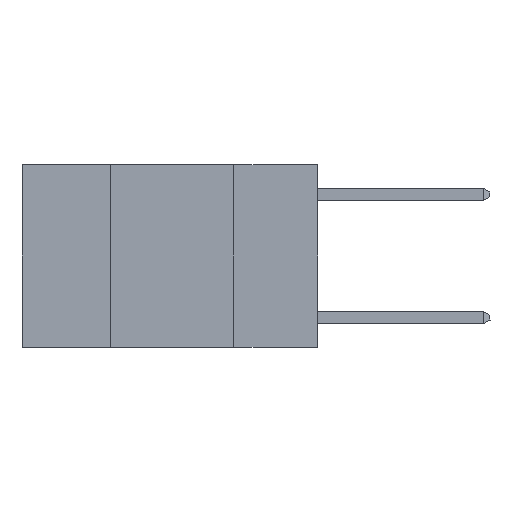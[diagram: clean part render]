
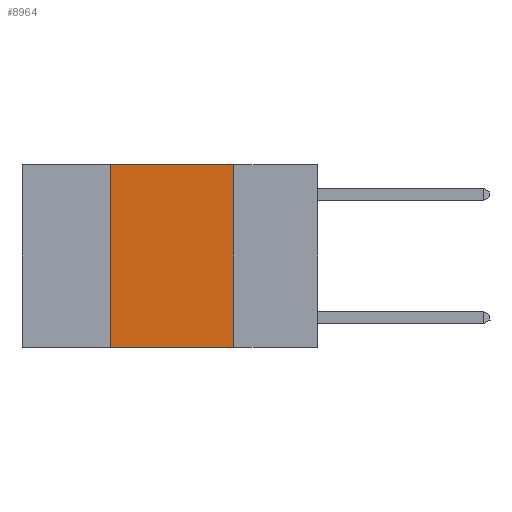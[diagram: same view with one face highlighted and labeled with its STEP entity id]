
A CAD part, left-side view. The second image highlights one B-rep face of the part: STEP entity #8964.
In plain terms, the highlighted planar face has unit normal (-1, 0, 0).
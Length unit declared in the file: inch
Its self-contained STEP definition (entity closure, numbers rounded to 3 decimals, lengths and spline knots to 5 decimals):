
#410 = VECTOR ( 'NONE', #20611, 39.37008 ) ;
#886 = CARTESIAN_POINT ( 'NONE',  ( 0., 0.42, 0. ) ) ;
#2584 = PLANE ( 'NONE',  #5424 ) ;
#3542 = VERTEX_POINT ( 'NONE', #16980 ) ;
#3792 = ORIENTED_EDGE ( 'NONE', *, *, #15846, .F. ) ;
#4309 = ORIENTED_EDGE ( 'NONE', *, *, #14849, .F. ) ;
#4364 = ORIENTED_EDGE ( 'NONE', *, *, #19608, .F. ) ;
#4509 = EDGE_LOOP ( 'NONE', ( #3792, #4309, #4364, #4764 ) ) ;
#4635 = CARTESIAN_POINT ( 'NONE',  ( 0., 0.6, 0. ) ) ;
#4764 = ORIENTED_EDGE ( 'NONE', *, *, #20805, .T. ) ;
#5039 = LINE ( 'NONE', #11954, #9811 ) ;
#5085 = VERTEX_POINT ( 'NONE', #16640 ) ;
#5424 = AXIS2_PLACEMENT_3D ( 'NONE', #4635, #18350, #6670 ) ;
#5779 = LINE ( 'NONE', #15813, #15697 ) ;
#6670 = DIRECTION ( 'NONE',  ( 0., 0., -1. ) ) ;
#6829 = VERTEX_POINT ( 'NONE', #14245 ) ;
#7136 = CARTESIAN_POINT ( 'NONE',  ( 0., 0.6, 0. ) ) ;
#8964 = ADVANCED_FACE ( 'NONE', ( #15971 ), #2584, .F. ) ;
#9811 = VECTOR ( 'NONE', #17681, 39.37008 ) ;
#10138 = DIRECTION ( 'NONE',  ( 0., -1., 0. ) ) ;
#11185 = LINE ( 'NONE', #7136, #410 ) ;
#11954 = CARTESIAN_POINT ( 'NONE',  ( 0., 0.17, 0. ) ) ;
#12694 = LINE ( 'NONE', #21496, #22035 ) ;
#14245 = CARTESIAN_POINT ( 'NONE',  ( 0., 0.17, -0.37 ) ) ;
#14849 = EDGE_CURVE ( 'NONE', #17835, #5085, #11185, .T. ) ;
#15697 = VECTOR ( 'NONE', #24899, 39.37008 ) ;
#15813 = CARTESIAN_POINT ( 'NONE',  ( 0., 0.42, 0. ) ) ;
#15846 = EDGE_CURVE ( 'NONE', #5085, #6829, #5039, .T. ) ;
#15971 = FACE_OUTER_BOUND ( 'NONE', #4509, .T. ) ;
#16640 = CARTESIAN_POINT ( 'NONE',  ( 0., 0.17, 0. ) ) ;
#16980 = CARTESIAN_POINT ( 'NONE',  ( 0., 0.42, -0.37 ) ) ;
#17681 = DIRECTION ( 'NONE',  ( 0., 0., -1. ) ) ;
#17835 = VERTEX_POINT ( 'NONE', #886 ) ;
#18350 = DIRECTION ( 'NONE',  ( 1., 0., 0. ) ) ;
#19608 = EDGE_CURVE ( 'NONE', #3542, #17835, #5779, .T. ) ;
#20611 = DIRECTION ( 'NONE',  ( 0., -1., 0. ) ) ;
#20805 = EDGE_CURVE ( 'NONE', #3542, #6829, #12694, .T. ) ;
#21496 = CARTESIAN_POINT ( 'NONE',  ( 0., 0.6, -0.37 ) ) ;
#22035 = VECTOR ( 'NONE', #10138, 39.37008 ) ;
#24899 = DIRECTION ( 'NONE',  ( 0., 0., 1. ) ) ;
